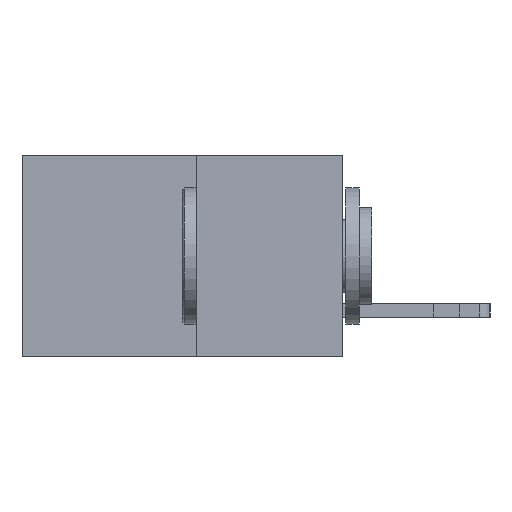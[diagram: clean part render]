
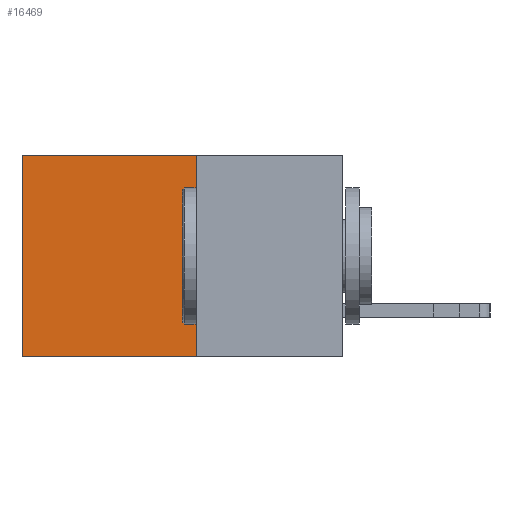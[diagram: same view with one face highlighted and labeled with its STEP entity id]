
A CAD part, left-side view. The second image highlights one B-rep face of the part: STEP entity #16469.
In plain terms, the highlighted planar face has unit normal (-1, 0, 0).
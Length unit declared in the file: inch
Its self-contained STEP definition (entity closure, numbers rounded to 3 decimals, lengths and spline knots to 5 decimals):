
#979 = EDGE_CURVE ( 'NONE', #12252, #2421, #4239, .T. ) ;
#1101 = VECTOR ( 'NONE', #10662, 39.37008 ) ;
#2064 = CARTESIAN_POINT ( 'NONE',  ( 0.277, 0.27, 0. ) ) ;
#2421 = VERTEX_POINT ( 'NONE', #12889 ) ;
#2893 = EDGE_CURVE ( 'NONE', #9562, #12252, #14206, .T. ) ;
#4127 = EDGE_CURVE ( 'NONE', #9562, #4198, #5357, .T. ) ;
#4198 = VERTEX_POINT ( 'NONE', #9761 ) ;
#4239 = LINE ( 'NONE', #15153, #13731 ) ;
#4532 = DIRECTION ( 'NONE',  ( 1., 0., 0. ) ) ;
#4696 = CARTESIAN_POINT ( 'NONE',  ( 0.277, 0.27, -0.37 ) ) ;
#4851 = EDGE_CURVE ( 'NONE', #4198, #2421, #15616, .T. ) ;
#5269 = ORIENTED_EDGE ( 'NONE', *, *, #4127, .T. ) ;
#5357 = LINE ( 'NONE', #10710, #1101 ) ;
#5787 = VECTOR ( 'NONE', #10124, 39.37008 ) ;
#7191 = EDGE_LOOP ( 'NONE', ( #7882, #11227, #10485, #5269 ) ) ;
#7383 = DIRECTION ( 'NONE',  ( 0., 1., 0. ) ) ;
#7882 = ORIENTED_EDGE ( 'NONE', *, *, #4851, .T. ) ;
#9562 = VERTEX_POINT ( 'NONE', #2064 ) ;
#9665 = CARTESIAN_POINT ( 'NONE',  ( 0.277, 0.27, -0.37 ) ) ;
#9761 = CARTESIAN_POINT ( 'NONE',  ( 0.277, 0.59, 0. ) ) ;
#9998 = VECTOR ( 'NONE', #12965, 39.37008 ) ;
#10124 = DIRECTION ( 'NONE',  ( 0., 0., -1. ) ) ;
#10139 = CARTESIAN_POINT ( 'NONE',  ( 0.277, 0.59, -0.37 ) ) ;
#10485 = ORIENTED_EDGE ( 'NONE', *, *, #2893, .F. ) ;
#10662 = DIRECTION ( 'NONE',  ( 0., 1., 0. ) ) ;
#10710 = CARTESIAN_POINT ( 'NONE',  ( 0.277, 0.27, 0. ) ) ;
#11227 = ORIENTED_EDGE ( 'NONE', *, *, #979, .F. ) ;
#12252 = VERTEX_POINT ( 'NONE', #4696 ) ;
#12647 = CARTESIAN_POINT ( 'NONE',  ( 0.277, 0.27, -0.37 ) ) ;
#12889 = CARTESIAN_POINT ( 'NONE',  ( 0.277, 0.59, -0.37 ) ) ;
#12965 = DIRECTION ( 'NONE',  ( 0., 0., -1. ) ) ;
#13524 = DIRECTION ( 'NONE',  ( 0., 0., -1. ) ) ;
#13731 = VECTOR ( 'NONE', #7383, 39.37008 ) ;
#14057 = FACE_OUTER_BOUND ( 'NONE', #7191, .T. ) ;
#14060 = AXIS2_PLACEMENT_3D ( 'NONE', #9665, #4532, #13524 ) ;
#14206 = LINE ( 'NONE', #12647, #9998 ) ;
#14724 = PLANE ( 'NONE',  #14060 ) ;
#15153 = CARTESIAN_POINT ( 'NONE',  ( 0.277, 0.27, -0.37 ) ) ;
#15616 = LINE ( 'NONE', #10139, #5787 ) ;
#16469 = ADVANCED_FACE ( 'NONE', ( #14057 ), #14724, .F. ) ;
